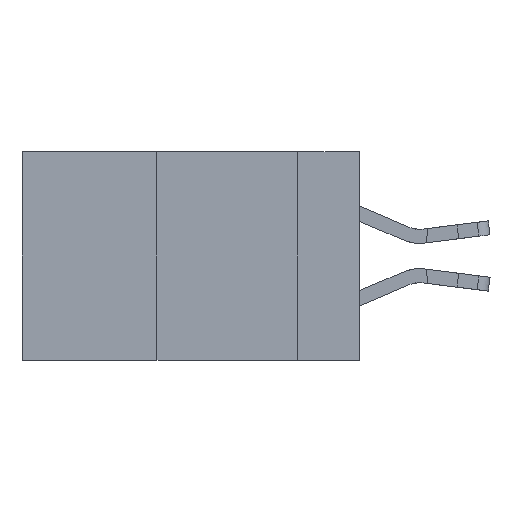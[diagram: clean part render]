
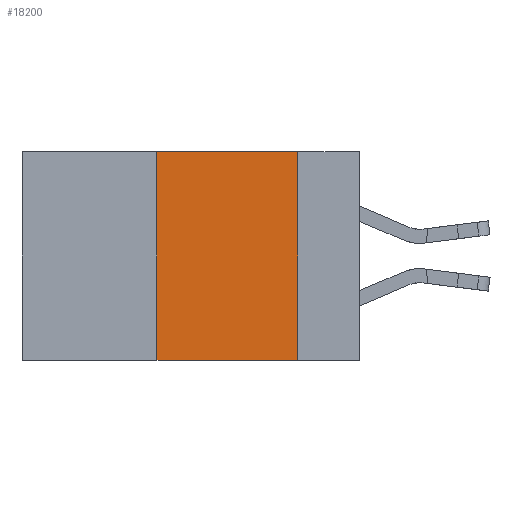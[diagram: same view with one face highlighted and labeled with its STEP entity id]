
A CAD part, left-side view. The second image highlights one B-rep face of the part: STEP entity #18200.
In plain terms, the highlighted planar face has unit normal (-1, 0, 0).
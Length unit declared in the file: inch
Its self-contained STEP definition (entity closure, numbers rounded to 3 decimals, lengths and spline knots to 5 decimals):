
#1071 = VERTEX_POINT ( 'NONE', #24687 ) ;
#1195 = DIRECTION ( 'NONE',  ( 0., 0., 1. ) ) ;
#1303 = CARTESIAN_POINT ( 'NONE',  ( 0., 0.6, 0. ) ) ;
#3583 = VERTEX_POINT ( 'NONE', #15194 ) ;
#3955 = DIRECTION ( 'NONE',  ( 0., 0., -1. ) ) ;
#3978 = CARTESIAN_POINT ( 'NONE',  ( 0., 0.6, -0.37 ) ) ;
#4314 = CARTESIAN_POINT ( 'NONE',  ( 0., 0.11, 0. ) ) ;
#5598 = DIRECTION ( 'NONE',  ( 0., -1., 0. ) ) ;
#6192 = EDGE_CURVE ( 'NONE', #3583, #1071, #25338, .T. ) ;
#7369 = CARTESIAN_POINT ( 'NONE',  ( 0., 0.36, 0. ) ) ;
#7916 = DIRECTION ( 'NONE',  ( 0., -1., 0. ) ) ;
#8505 = EDGE_CURVE ( 'NONE', #21474, #11285, #13209, .T. ) ;
#8655 = VECTOR ( 'NONE', #1195, 39.37008 ) ;
#10321 = VECTOR ( 'NONE', #5598, 39.37008 ) ;
#10693 = CARTESIAN_POINT ( 'NONE',  ( 0., 0.11, 0. ) ) ;
#10765 = LINE ( 'NONE', #4314, #26627 ) ;
#11285 = VERTEX_POINT ( 'NONE', #10693 ) ;
#11521 = PLANE ( 'NONE',  #24608 ) ;
#13209 = LINE ( 'NONE', #26472, #10321 ) ;
#13885 = EDGE_CURVE ( 'NONE', #3583, #21474, #19913, .T. ) ;
#15194 = CARTESIAN_POINT ( 'NONE',  ( 0., 0.36, -0.37 ) ) ;
#15965 = EDGE_CURVE ( 'NONE', #11285, #1071, #10765, .T. ) ;
#17998 = EDGE_LOOP ( 'NONE', ( #20723, #18506, #20164, #19360 ) ) ;
#18200 = ADVANCED_FACE ( 'NONE', ( #19625 ), #11521, .F. ) ;
#18506 = ORIENTED_EDGE ( 'NONE', *, *, #8505, .F. ) ;
#19360 = ORIENTED_EDGE ( 'NONE', *, *, #6192, .T. ) ;
#19625 = FACE_OUTER_BOUND ( 'NONE', #17998, .T. ) ;
#19648 = CARTESIAN_POINT ( 'NONE',  ( 0., 0.36, 0. ) ) ;
#19913 = LINE ( 'NONE', #7369, #8655 ) ;
#20164 = ORIENTED_EDGE ( 'NONE', *, *, #13885, .F. ) ;
#20723 = ORIENTED_EDGE ( 'NONE', *, *, #15965, .F. ) ;
#21474 = VERTEX_POINT ( 'NONE', #19648 ) ;
#21927 = DIRECTION ( 'NONE',  ( 1., 0., 0. ) ) ;
#22101 = VECTOR ( 'NONE', #7916, 39.37008 ) ;
#23737 = DIRECTION ( 'NONE',  ( 0., 0., -1. ) ) ;
#24608 = AXIS2_PLACEMENT_3D ( 'NONE', #1303, #21927, #23737 ) ;
#24687 = CARTESIAN_POINT ( 'NONE',  ( 0., 0.11, -0.37 ) ) ;
#25338 = LINE ( 'NONE', #3978, #22101 ) ;
#26472 = CARTESIAN_POINT ( 'NONE',  ( 0., 0.6, 0. ) ) ;
#26627 = VECTOR ( 'NONE', #3955, 39.37008 ) ;
